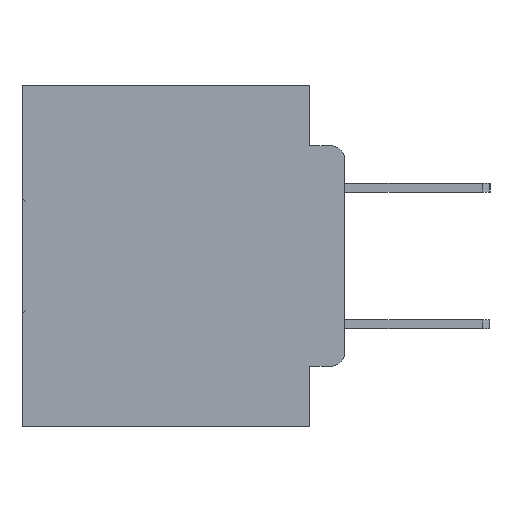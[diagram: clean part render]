
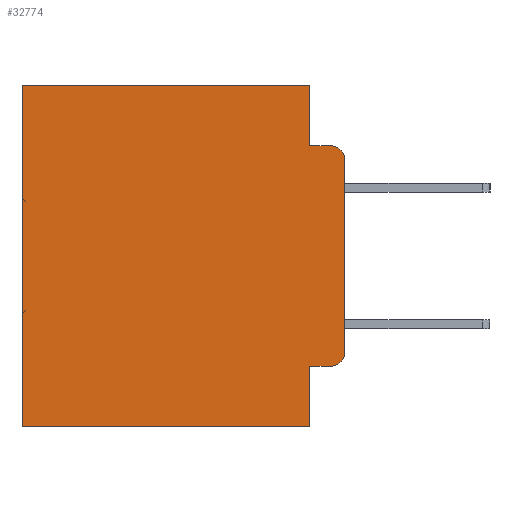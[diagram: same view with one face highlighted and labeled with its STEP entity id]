
A CAD part, left-side view. The second image highlights one B-rep face of the part: STEP entity #32774.
In plain terms, the highlighted planar face has unit normal (-1, 0, 0).
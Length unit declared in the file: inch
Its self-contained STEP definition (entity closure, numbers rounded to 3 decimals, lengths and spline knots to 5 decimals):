
#371 = DIRECTION ( 'NONE',  ( 0., 0., -1. ) ) ;
#373 = CIRCLE ( 'NONE', #26501, 0.02 ) ;
#638 = LINE ( 'NONE', #20916, #14585 ) ;
#1149 = LINE ( 'NONE', #25856, #33150 ) ;
#1237 = DIRECTION ( 'NONE',  ( 0., 0., -1. ) ) ;
#1337 = ORIENTED_EDGE ( 'NONE', *, *, #29066, .F. ) ;
#1488 = CARTESIAN_POINT ( 'NONE',  ( 0.298, 0.02, -0.3915 ) ) ;
#1657 = DIRECTION ( 'NONE',  ( -1., 0., 0. ) ) ;
#2231 = EDGE_CURVE ( 'NONE', #24609, #31252, #373, .T. ) ;
#2627 = DIRECTION ( 'NONE',  ( 0., -1., 0. ) ) ;
#2686 = DIRECTION ( 'NONE',  ( 0., 0., -1. ) ) ;
#3400 = ORIENTED_EDGE ( 'NONE', *, *, #8931, .T. ) ;
#3483 = CARTESIAN_POINT ( 'NONE',  ( 0.298, 0.051, -0.0885 ) ) ;
#4666 = ORIENTED_EDGE ( 'NONE', *, *, #12282, .T. ) ;
#5001 = ORIENTED_EDGE ( 'NONE', *, *, #8264, .T. ) ;
#5201 = VECTOR ( 'NONE', #21746, 39.37008 ) ;
#5367 = VERTEX_POINT ( 'NONE', #24746 ) ;
#5682 = CARTESIAN_POINT ( 'NONE',  ( 0.298, 0.051, -0.0885 ) ) ;
#6574 = VERTEX_POINT ( 'NONE', #5682 ) ;
#6814 = LINE ( 'NONE', #10658, #26387 ) ;
#8150 = CARTESIAN_POINT ( 'NONE',  ( 0.298, 0.051, 0. ) ) ;
#8264 = EDGE_CURVE ( 'NONE', #31585, #5367, #6814, .T. ) ;
#8274 = VERTEX_POINT ( 'NONE', #18441 ) ;
#8394 = VERTEX_POINT ( 'NONE', #8433 ) ;
#8433 = CARTESIAN_POINT ( 'NONE',  ( 0.298, 0.02, -0.0885 ) ) ;
#8931 = EDGE_CURVE ( 'NONE', #28905, #24609, #638, .T. ) ;
#9307 = AXIS2_PLACEMENT_3D ( 'NONE', #10928, #28958, #13512 ) ;
#9866 = ORIENTED_EDGE ( 'NONE', *, *, #18052, .F. ) ;
#10555 = DIRECTION ( 'NONE',  ( -1., 0., 0. ) ) ;
#10658 = CARTESIAN_POINT ( 'NONE',  ( 0.298, 0., 0. ) ) ;
#10928 = CARTESIAN_POINT ( 'NONE',  ( 0.298, 0., 0. ) ) ;
#11192 = ORIENTED_EDGE ( 'NONE', *, *, #27937, .F. ) ;
#11455 = LINE ( 'NONE', #14323, #17478 ) ;
#11675 = CARTESIAN_POINT ( 'NONE',  ( 0.298, 0., -0.5 ) ) ;
#11957 = VECTOR ( 'NONE', #2686, 39.37008 ) ;
#12281 = FACE_OUTER_BOUND ( 'NONE', #18135, .T. ) ;
#12282 = EDGE_CURVE ( 'NONE', #8274, #8394, #29306, .T. ) ;
#13512 = DIRECTION ( 'NONE',  ( 0., 0., -1. ) ) ;
#13690 = ORIENTED_EDGE ( 'NONE', *, *, #27613, .F. ) ;
#14323 = CARTESIAN_POINT ( 'NONE',  ( 0.298, 0., 0. ) ) ;
#14585 = VECTOR ( 'NONE', #2627, 39.37008 ) ;
#16212 = VECTOR ( 'NONE', #29701, 39.37008 ) ;
#16521 = VERTEX_POINT ( 'NONE', #17771 ) ;
#17182 = LINE ( 'NONE', #18341, #11957 ) ;
#17478 = VECTOR ( 'NONE', #1237, 39.37008 ) ;
#17771 = CARTESIAN_POINT ( 'NONE',  ( 0.298, 0.473, -0.5 ) ) ;
#17956 = EDGE_CURVE ( 'NONE', #31585, #6574, #21554, .T. ) ;
#18052 = EDGE_CURVE ( 'NONE', #6574, #8394, #31949, .T. ) ;
#18135 = EDGE_LOOP ( 'NONE', ( #11192, #4666, #9866, #18639, #5001, #33372, #1337, #13690, #3400, #22577 ) ) ;
#18341 = CARTESIAN_POINT ( 'NONE',  ( 0.298, 0.473, 0. ) ) ;
#18441 = CARTESIAN_POINT ( 'NONE',  ( 0.298, 0., -0.1085 ) ) ;
#18639 = ORIENTED_EDGE ( 'NONE', *, *, #17956, .F. ) ;
#20739 = VECTOR ( 'NONE', #21114, 39.37008 ) ;
#20916 = CARTESIAN_POINT ( 'NONE',  ( 0.298, 0.051, -0.4115 ) ) ;
#21114 = DIRECTION ( 'NONE',  ( 0., 0., -1. ) ) ;
#21554 = LINE ( 'NONE', #8150, #20739 ) ;
#21746 = DIRECTION ( 'NONE',  ( 0., -1., 0. ) ) ;
#22577 = ORIENTED_EDGE ( 'NONE', *, *, #2231, .T. ) ;
#23021 = CARTESIAN_POINT ( 'NONE',  ( 0.298, 0.051, 0. ) ) ;
#23050 = AXIS2_PLACEMENT_3D ( 'NONE', #26035, #10555, #28606 ) ;
#23070 = CARTESIAN_POINT ( 'NONE',  ( 0.298, 0.02, -0.4115 ) ) ;
#23093 = LINE ( 'NONE', #11675, #16212 ) ;
#23906 = CARTESIAN_POINT ( 'NONE',  ( 0.298, 0.051, -0.4115 ) ) ;
#24118 = VERTEX_POINT ( 'NONE', #28470 ) ;
#24609 = VERTEX_POINT ( 'NONE', #23070 ) ;
#24746 = CARTESIAN_POINT ( 'NONE',  ( 0.298, 0.473, 0. ) ) ;
#25856 = CARTESIAN_POINT ( 'NONE',  ( 0.298, 0.051, 0. ) ) ;
#26035 = CARTESIAN_POINT ( 'NONE',  ( 0.298, 0.02, -0.1085 ) ) ;
#26128 = DIRECTION ( 'NONE',  ( 0., 1., 0. ) ) ;
#26387 = VECTOR ( 'NONE', #26128, 39.37008 ) ;
#26409 = PLANE ( 'NONE',  #9307 ) ;
#26501 = AXIS2_PLACEMENT_3D ( 'NONE', #1488, #1657, #371 ) ;
#26861 = CARTESIAN_POINT ( 'NONE',  ( 0.298, 0., -0.3915 ) ) ;
#27613 = EDGE_CURVE ( 'NONE', #28905, #24118, #1149, .T. ) ;
#27937 = EDGE_CURVE ( 'NONE', #8274, #31252, #11455, .T. ) ;
#28441 = DIRECTION ( 'NONE',  ( 0., 0., -1. ) ) ;
#28470 = CARTESIAN_POINT ( 'NONE',  ( 0.298, 0.051, -0.5 ) ) ;
#28606 = DIRECTION ( 'NONE',  ( 0., 0., -1. ) ) ;
#28905 = VERTEX_POINT ( 'NONE', #23906 ) ;
#28958 = DIRECTION ( 'NONE',  ( 1., 0., 0. ) ) ;
#29066 = EDGE_CURVE ( 'NONE', #24118, #16521, #23093, .T. ) ;
#29306 = CIRCLE ( 'NONE', #23050, 0.02 ) ;
#29701 = DIRECTION ( 'NONE',  ( 0., 1., 0. ) ) ;
#31252 = VERTEX_POINT ( 'NONE', #26861 ) ;
#31585 = VERTEX_POINT ( 'NONE', #23021 ) ;
#31714 = EDGE_CURVE ( 'NONE', #5367, #16521, #17182, .T. ) ;
#31949 = LINE ( 'NONE', #3483, #5201 ) ;
#32774 = ADVANCED_FACE ( 'NONE', ( #12281 ), #26409, .F. ) ;
#33150 = VECTOR ( 'NONE', #28441, 39.37008 ) ;
#33372 = ORIENTED_EDGE ( 'NONE', *, *, #31714, .T. ) ;
